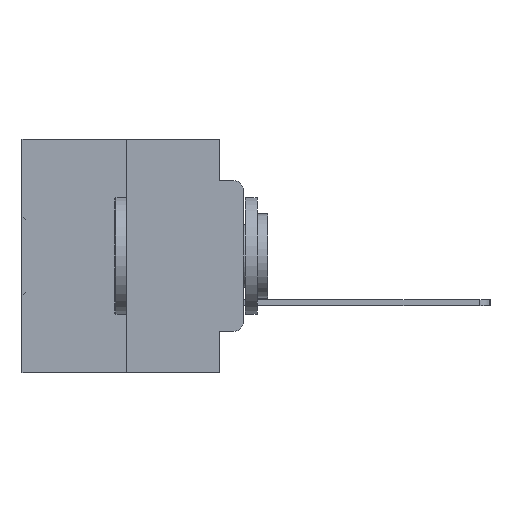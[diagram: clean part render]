
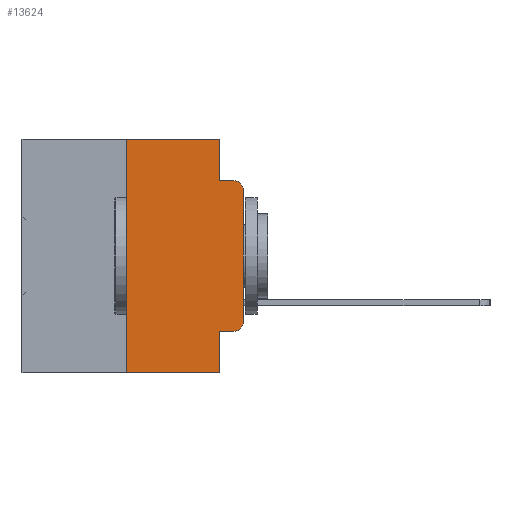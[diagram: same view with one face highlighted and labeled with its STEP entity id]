
A CAD part, left-side view. The second image highlights one B-rep face of the part: STEP entity #13624.
In plain terms, the highlighted planar face has unit normal (-1, 0, 0).
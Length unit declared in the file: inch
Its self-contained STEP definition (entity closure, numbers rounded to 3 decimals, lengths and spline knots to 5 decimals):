
#241 = AXIS2_PLACEMENT_3D ( 'NONE', #16672, #622, #19239 ) ;
#320 = ORIENTED_EDGE ( 'NONE', *, *, #21390, .T. ) ;
#453 = CARTESIAN_POINT ( 'NONE',  ( 0., 0., 0. ) ) ;
#610 = VERTEX_POINT ( 'NONE', #14039 ) ;
#622 = DIRECTION ( 'NONE',  ( -1., 0., 0. ) ) ;
#781 = CARTESIAN_POINT ( 'NONE',  ( 0., 0.473, -0.5 ) ) ;
#820 = CARTESIAN_POINT ( 'NONE',  ( 0., 0.051, -0.4115 ) ) ;
#880 = ORIENTED_EDGE ( 'NONE', *, *, #17984, .T. ) ;
#1055 = CARTESIAN_POINT ( 'NONE',  ( 0., 0.473, 0. ) ) ;
#1213 = EDGE_CURVE ( 'NONE', #13807, #3049, #26115, .T. ) ;
#1678 = VERTEX_POINT ( 'NONE', #26436 ) ;
#1841 = CARTESIAN_POINT ( 'NONE',  ( 0., 0.473, 0. ) ) ;
#2207 = VECTOR ( 'NONE', #8313, 39.37008 ) ;
#2778 = VERTEX_POINT ( 'NONE', #7347 ) ;
#2875 = VERTEX_POINT ( 'NONE', #24030 ) ;
#3049 = VERTEX_POINT ( 'NONE', #24697 ) ;
#3204 = LINE ( 'NONE', #781, #10396 ) ;
#3369 = CIRCLE ( 'NONE', #241, 0.02 ) ;
#3833 = DIRECTION ( 'NONE',  ( 0., -1., 0. ) ) ;
#4720 = PLANE ( 'NONE',  #26081 ) ;
#5184 = AXIS2_PLACEMENT_3D ( 'NONE', #29135, #13657, #31752 ) ;
#5313 = VECTOR ( 'NONE', #19415, 39.37008 ) ;
#5550 = EDGE_LOOP ( 'NONE', ( #7770, #21785, #22861, #14803, #11050, #7830, #6173, #9609, #320, #880 ) ) ;
#5576 = VECTOR ( 'NONE', #31105, 39.37008 ) ;
#6173 = ORIENTED_EDGE ( 'NONE', *, *, #20111, .T. ) ;
#6257 = DIRECTION ( 'NONE',  ( 0., -1., 0. ) ) ;
#6564 = CARTESIAN_POINT ( 'NONE',  ( 0., 0.25, 0. ) ) ;
#7347 = CARTESIAN_POINT ( 'NONE',  ( 0., 0.25, -0.5 ) ) ;
#7475 = DIRECTION ( 'NONE',  ( 1., 0., 0. ) ) ;
#7642 = VECTOR ( 'NONE', #6257, 39.37008 ) ;
#7770 = ORIENTED_EDGE ( 'NONE', *, *, #1213, .T. ) ;
#7830 = ORIENTED_EDGE ( 'NONE', *, *, #24854, .F. ) ;
#8313 = DIRECTION ( 'NONE',  ( 0., 0., -1. ) ) ;
#9443 = LINE ( 'NONE', #26389, #2207 ) ;
#9609 = ORIENTED_EDGE ( 'NONE', *, *, #23113, .F. ) ;
#9927 = CARTESIAN_POINT ( 'NONE',  ( 0., 0.25, 0. ) ) ;
#10112 = CARTESIAN_POINT ( 'NONE',  ( 0., 0.02, -0.4115 ) ) ;
#10372 = CARTESIAN_POINT ( 'NONE',  ( 0., 0.051, 0. ) ) ;
#10396 = VECTOR ( 'NONE', #29687, 39.37008 ) ;
#11050 = ORIENTED_EDGE ( 'NONE', *, *, #21443, .F. ) ;
#11550 = LINE ( 'NONE', #820, #5313 ) ;
#12342 = VERTEX_POINT ( 'NONE', #10112 ) ;
#12551 = LINE ( 'NONE', #6564, #34017 ) ;
#13624 = ADVANCED_FACE ( 'NONE', ( #16508 ), #4720, .F. ) ;
#13657 = DIRECTION ( 'NONE',  ( -1., 0., 0. ) ) ;
#13807 = VERTEX_POINT ( 'NONE', #16084 ) ;
#13889 = DIRECTION ( 'NONE',  ( 0., 0., 1. ) ) ;
#14039 = CARTESIAN_POINT ( 'NONE',  ( 0., 0.051, -0.5 ) ) ;
#14157 = CARTESIAN_POINT ( 'NONE',  ( 0., 0.051, -0.0885 ) ) ;
#14623 = LINE ( 'NONE', #14157, #7642 ) ;
#14803 = ORIENTED_EDGE ( 'NONE', *, *, #26634, .F. ) ;
#15137 = LINE ( 'NONE', #10372, #5576 ) ;
#16084 = CARTESIAN_POINT ( 'NONE',  ( 0., 0., -0.3915 ) ) ;
#16508 = FACE_OUTER_BOUND ( 'NONE', #5550, .T. ) ;
#16672 = CARTESIAN_POINT ( 'NONE',  ( 0., 0.02, -0.3915 ) ) ;
#16886 = VECTOR ( 'NONE', #3833, 39.37008 ) ;
#17436 = CARTESIAN_POINT ( 'NONE',  ( 0., 0.051, -0.4115 ) ) ;
#17701 = LINE ( 'NONE', #1055, #16886 ) ;
#17984 = EDGE_CURVE ( 'NONE', #12342, #13807, #3369, .T. ) ;
#19239 = DIRECTION ( 'NONE',  ( 0., 0., -1. ) ) ;
#19415 = DIRECTION ( 'NONE',  ( 0., -1., 0. ) ) ;
#20111 = EDGE_CURVE ( 'NONE', #2778, #610, #3204, .T. ) ;
#21390 = EDGE_CURVE ( 'NONE', #23470, #12342, #11550, .T. ) ;
#21443 = EDGE_CURVE ( 'NONE', #31005, #32056, #17701, .T. ) ;
#21785 = ORIENTED_EDGE ( 'NONE', *, *, #30076, .T. ) ;
#22187 = DIRECTION ( 'NONE',  ( 0., 0., 1. ) ) ;
#22861 = ORIENTED_EDGE ( 'NONE', *, *, #28362, .F. ) ;
#23113 = EDGE_CURVE ( 'NONE', #23470, #610, #15137, .T. ) ;
#23470 = VERTEX_POINT ( 'NONE', #17436 ) ;
#24030 = CARTESIAN_POINT ( 'NONE',  ( 0., 0.02, -0.0885 ) ) ;
#24697 = CARTESIAN_POINT ( 'NONE',  ( 0., 0., -0.1085 ) ) ;
#24813 = CARTESIAN_POINT ( 'NONE',  ( 0., 0.051, 0. ) ) ;
#24854 = EDGE_CURVE ( 'NONE', #2778, #31005, #12551, .T. ) ;
#25677 = DIRECTION ( 'NONE',  ( 0., 0., -1. ) ) ;
#26081 = AXIS2_PLACEMENT_3D ( 'NONE', #1841, #7475, #25677 ) ;
#26115 = LINE ( 'NONE', #453, #32164 ) ;
#26389 = CARTESIAN_POINT ( 'NONE',  ( 0., 0.051, 0. ) ) ;
#26436 = CARTESIAN_POINT ( 'NONE',  ( 0., 0.051, -0.0885 ) ) ;
#26634 = EDGE_CURVE ( 'NONE', #32056, #1678, #9443, .T. ) ;
#28362 = EDGE_CURVE ( 'NONE', #1678, #2875, #14623, .T. ) ;
#29002 = CIRCLE ( 'NONE', #5184, 0.02 ) ;
#29135 = CARTESIAN_POINT ( 'NONE',  ( 0., 0.02, -0.1085 ) ) ;
#29687 = DIRECTION ( 'NONE',  ( 0., -1., 0. ) ) ;
#30076 = EDGE_CURVE ( 'NONE', #3049, #2875, #29002, .T. ) ;
#31005 = VERTEX_POINT ( 'NONE', #9927 ) ;
#31105 = DIRECTION ( 'NONE',  ( 0., 0., -1. ) ) ;
#31752 = DIRECTION ( 'NONE',  ( 0., 0., -1. ) ) ;
#32056 = VERTEX_POINT ( 'NONE', #24813 ) ;
#32164 = VECTOR ( 'NONE', #13889, 39.37008 ) ;
#34017 = VECTOR ( 'NONE', #22187, 39.37008 ) ;
